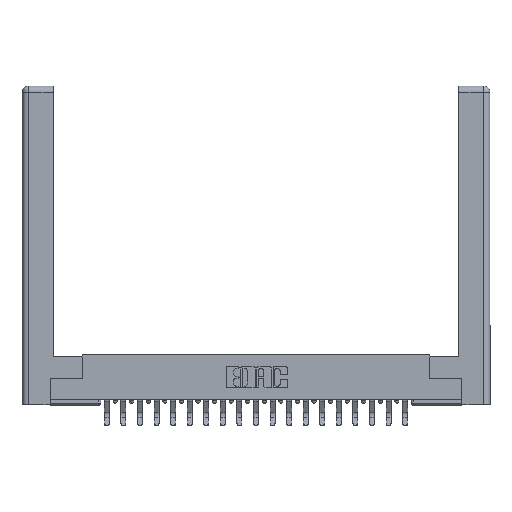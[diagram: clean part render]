
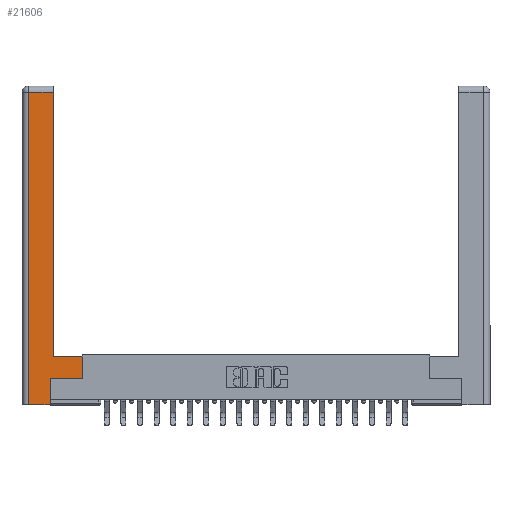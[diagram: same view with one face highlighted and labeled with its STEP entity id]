
A CAD part, top view. The second image highlights one B-rep face of the part: STEP entity #21606.
In plain terms, the highlighted planar face has unit normal (0, 0, 1).
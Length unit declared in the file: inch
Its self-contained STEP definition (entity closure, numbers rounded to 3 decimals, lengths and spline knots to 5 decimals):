
#686 = DIRECTION ( 'NONE',  ( 0., 1., 0. ) ) ;
#813 = VERTEX_POINT ( 'NONE', #6766 ) ;
#998 = DIRECTION ( 'NONE',  ( 0., 0., -1. ) ) ;
#1818 = VECTOR ( 'NONE', #15986, 39.37008 ) ;
#1939 = LINE ( 'NONE', #10829, #17656 ) ;
#2109 = VERTEX_POINT ( 'NONE', #20805 ) ;
#2448 = LINE ( 'NONE', #3255, #4873 ) ;
#2470 = VERTEX_POINT ( 'NONE', #4373 ) ;
#3255 = CARTESIAN_POINT ( 'NONE',  ( 0.565, 0.45, 0. ) ) ;
#3484 = CARTESIAN_POINT ( 'NONE',  ( 0.565, 0.245, 0. ) ) ;
#4133 = VECTOR ( 'NONE', #19907, 39.37008 ) ;
#4373 = CARTESIAN_POINT ( 'NONE',  ( 0.295, 0.45, 0. ) ) ;
#4873 = VECTOR ( 'NONE', #10457, 39.37008 ) ;
#4911 = VERTEX_POINT ( 'NONE', #9357 ) ;
#5838 = EDGE_CURVE ( 'NONE', #14705, #4911, #22312, .T. ) ;
#6123 = VECTOR ( 'NONE', #17992, 39.37008 ) ;
#6239 = LINE ( 'NONE', #21472, #17071 ) ;
#6766 = CARTESIAN_POINT ( 'NONE',  ( 0.265, 0., 0. ) ) ;
#7405 = DIRECTION ( 'NONE',  ( 0., 1., 0. ) ) ;
#7612 = CARTESIAN_POINT ( 'NONE',  ( 0.295, 0.45, 0. ) ) ;
#7753 = CARTESIAN_POINT ( 'NONE',  ( 0.0615, 2.94, 0. ) ) ;
#7818 = ORIENTED_EDGE ( 'NONE', *, *, #11869, .T. ) ;
#7891 = LINE ( 'NONE', #7753, #4133 ) ;
#8587 = LINE ( 'NONE', #7612, #19753 ) ;
#8770 = EDGE_CURVE ( 'NONE', #18537, #2470, #8587, .T. ) ;
#8918 = CARTESIAN_POINT ( 'NONE',  ( 0.265, 0., 0. ) ) ;
#9357 = CARTESIAN_POINT ( 'NONE',  ( 0.565, 0.245, 0. ) ) ;
#9503 = VERTEX_POINT ( 'NONE', #17671 ) ;
#10457 = DIRECTION ( 'NONE',  ( 0., 1., 0. ) ) ;
#10730 = LINE ( 'NONE', #11233, #6123 ) ;
#10829 = CARTESIAN_POINT ( 'NONE',  ( 0.295, 3., 0. ) ) ;
#10905 = EDGE_CURVE ( 'NONE', #2109, #9503, #7891, .T. ) ;
#11014 = AXIS2_PLACEMENT_3D ( 'NONE', #16679, #998, #19974 ) ;
#11029 = ORIENTED_EDGE ( 'NONE', *, *, #18798, .T. ) ;
#11233 = CARTESIAN_POINT ( 'NONE',  ( 0.0615, 0., 0. ) ) ;
#11239 = ORIENTED_EDGE ( 'NONE', *, *, #11407, .T. ) ;
#11407 = EDGE_CURVE ( 'NONE', #813, #14705, #6239, .T. ) ;
#11437 = CARTESIAN_POINT ( 'NONE',  ( 0.265, 0.245, 0. ) ) ;
#11590 = FACE_OUTER_BOUND ( 'NONE', #15237, .T. ) ;
#11596 = CARTESIAN_POINT ( 'NONE',  ( 0.565, 0.45, 0. ) ) ;
#11658 = ORIENTED_EDGE ( 'NONE', *, *, #10905, .T. ) ;
#11869 = EDGE_CURVE ( 'NONE', #4911, #18537, #2448, .T. ) ;
#11957 = DIRECTION ( 'NONE',  ( 1., 0., 0. ) ) ;
#13040 = ORIENTED_EDGE ( 'NONE', *, *, #15196, .T. ) ;
#13294 = ORIENTED_EDGE ( 'NONE', *, *, #21934, .T. ) ;
#14173 = VECTOR ( 'NONE', #11957, 39.37008 ) ;
#14456 = DIRECTION ( 'NONE',  ( -1., 0., 0. ) ) ;
#14705 = VERTEX_POINT ( 'NONE', #11437 ) ;
#14945 = PLANE ( 'NONE',  #11014 ) ;
#15196 = EDGE_CURVE ( 'NONE', #9503, #17655, #10730, .T. ) ;
#15237 = EDGE_LOOP ( 'NONE', ( #11029, #11658, #13040, #13294, #11239, #16579, #7818, #20844 ) ) ;
#15986 = DIRECTION ( 'NONE',  ( 1., 0., 0. ) ) ;
#16579 = ORIENTED_EDGE ( 'NONE', *, *, #5838, .T. ) ;
#16679 = CARTESIAN_POINT ( 'NONE',  ( 0., 0., 0. ) ) ;
#17071 = VECTOR ( 'NONE', #686, 39.37008 ) ;
#17655 = VERTEX_POINT ( 'NONE', #20966 ) ;
#17656 = VECTOR ( 'NONE', #7405, 39.37008 ) ;
#17671 = CARTESIAN_POINT ( 'NONE',  ( 0.0615, 2.94, 0. ) ) ;
#17992 = DIRECTION ( 'NONE',  ( 0., -1., 0. ) ) ;
#18537 = VERTEX_POINT ( 'NONE', #11596 ) ;
#18798 = EDGE_CURVE ( 'NONE', #2470, #2109, #1939, .T. ) ;
#19453 = LINE ( 'NONE', #8918, #1818 ) ;
#19753 = VECTOR ( 'NONE', #14456, 39.37008 ) ;
#19907 = DIRECTION ( 'NONE',  ( -1., 0., 0. ) ) ;
#19974 = DIRECTION ( 'NONE',  ( -1., 0., 0. ) ) ;
#20805 = CARTESIAN_POINT ( 'NONE',  ( 0.295, 2.94, 0. ) ) ;
#20844 = ORIENTED_EDGE ( 'NONE', *, *, #8770, .T. ) ;
#20966 = CARTESIAN_POINT ( 'NONE',  ( 0.0615, 0., 0. ) ) ;
#21472 = CARTESIAN_POINT ( 'NONE',  ( 0.265, 0.245, 0. ) ) ;
#21606 = ADVANCED_FACE ( 'NONE', ( #11590 ), #14945, .F. ) ;
#21934 = EDGE_CURVE ( 'NONE', #17655, #813, #19453, .T. ) ;
#22312 = LINE ( 'NONE', #3484, #14173 ) ;
